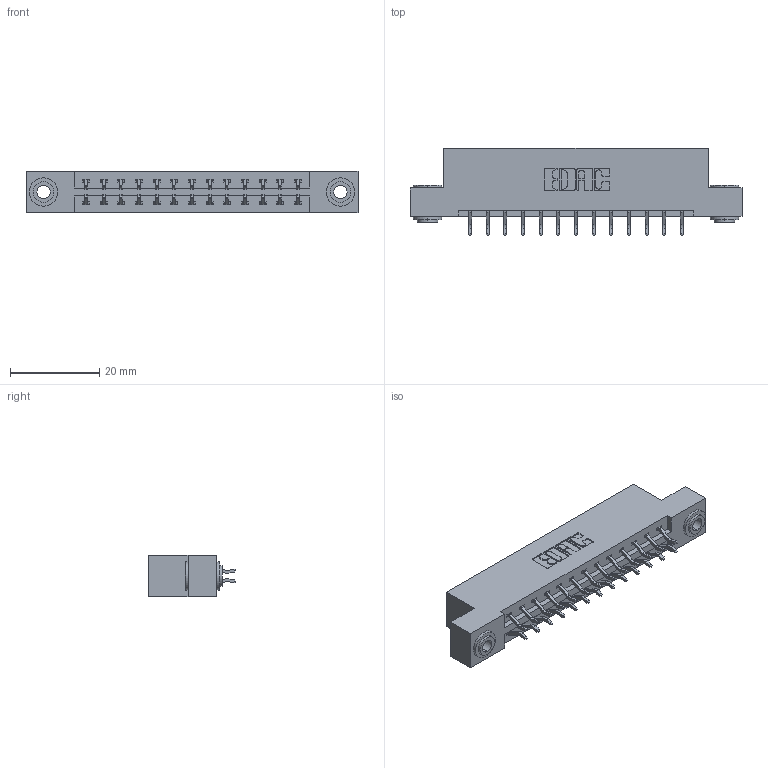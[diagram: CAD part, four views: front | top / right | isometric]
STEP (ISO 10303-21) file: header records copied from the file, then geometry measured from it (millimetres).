
FILE_DESCRIPTION (( 'STEP AP203' ), '1' );
FILE_NAME ('337-026-556-203.STEP', '2018-08-06T06:13:04', ( '' ), ( '' ), 'SwSTEP 2.0', 'SolidWorks 2016', '' );
FILE_SCHEMA (( 'CONFIG_CONTROL_DESIGN' ));
Length unit declared in the file: inch
Products named in the file (4): 345-292-001_556 Tail; 345-250-002_345-250-002-102; 337-026-556-203; 337 Part_Flush Mounting Lugs - 0.156 Dia-TH
Assembly tree (29 placements, depth 2):
  337-026-556-203
    337 Part_Flush Mounting Lugs - 0.156 Dia-TH
    345-292-001_556 Tail  x26
    345-250-002_345-250-002-102  x2
Bounding box: 74.52 x 19.57 x 9.4 mm (x, y, z)
Volume: 7486.2 mm3; surface area: 8378.5 mm2
Topology: 29 solids, 29 shells, 1712 faces, 5041 edges, 3322 vertices
Faces by surface type: plane 1172, cylinder 532, cone 8
Entity records: 14700 total; most frequent: CARTESIAN_POINT 2489, ORIENTED_EDGE 2406, DIRECTION 2193, EDGE_CURVE 1203, VECTOR 1043, LINE 1043, VERTEX_POINT 798, AXIS2_PLACEMENT_3D 575
